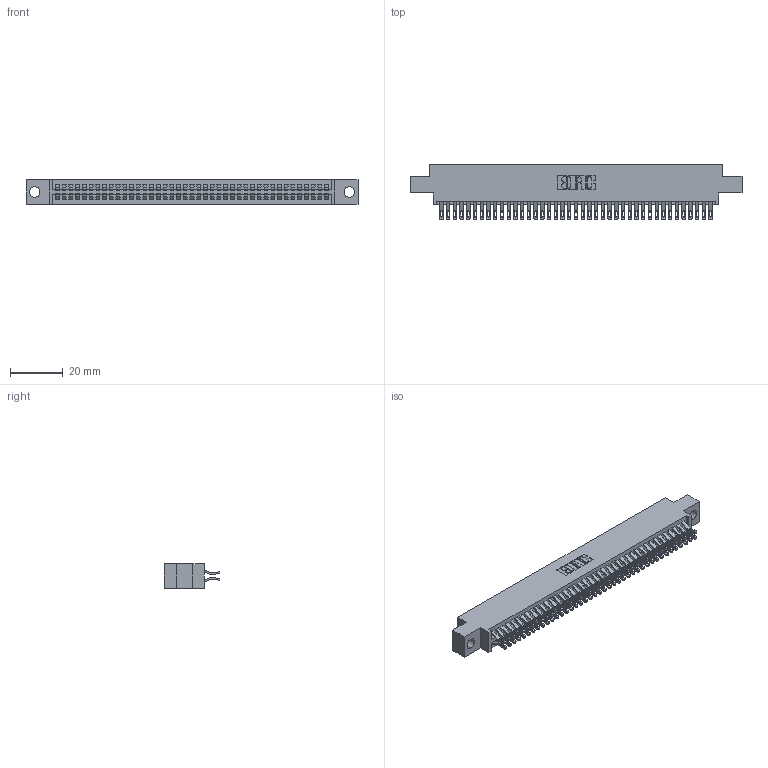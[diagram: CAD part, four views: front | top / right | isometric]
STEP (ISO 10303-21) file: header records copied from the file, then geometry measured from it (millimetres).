
FILE_DESCRIPTION (( 'STEP AP203' ), '1' );
FILE_NAME ('345-082-555-804.STEP', '2018-10-03T23:02:16', ( '' ), ( '' ), 'SwSTEP 2.0', 'SolidWorks 2016', '' );
FILE_SCHEMA (( 'CONFIG_CONTROL_DESIGN' ));
Length unit declared in the file: inch
Products named in the file (3): 345-292-001_555 Tail; 345-082-555-804; 345 Part_0.170 Offset - 0.156 Dia-TH
Assembly tree (83 placements, depth 2):
  345-082-555-804
    345 Part_0.170 Offset - 0.156 Dia-TH
    345-292-001_555 Tail  x82
Bounding box: 125.35 x 21.13 x 9.4 mm (x, y, z)
Volume: 12203.9 mm3; surface area: 18805.9 mm2
Topology: 83 solids, 83 shells, 4722 faces, 14867 edges, 9910 vertices
Faces by surface type: plane 2626, cylinder 2096
Entity records: 32765 total; most frequent: CARTESIAN_POINT 5530, ORIENTED_EDGE 5434, DIRECTION 4845, EDGE_CURVE 2717, VECTOR 2401, LINE 2401, VERTEX_POINT 1810, AXIS2_PLACEMENT_3D 1222
